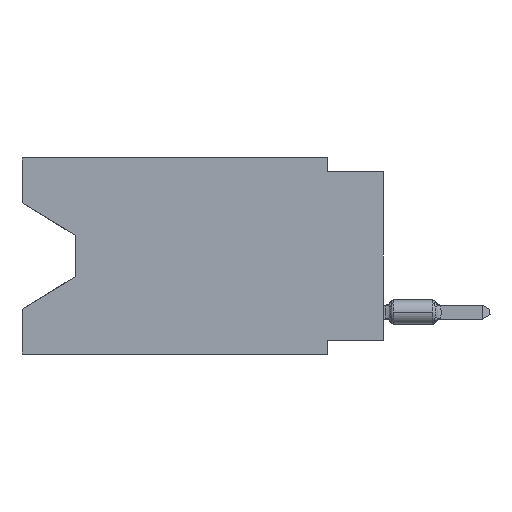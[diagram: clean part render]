
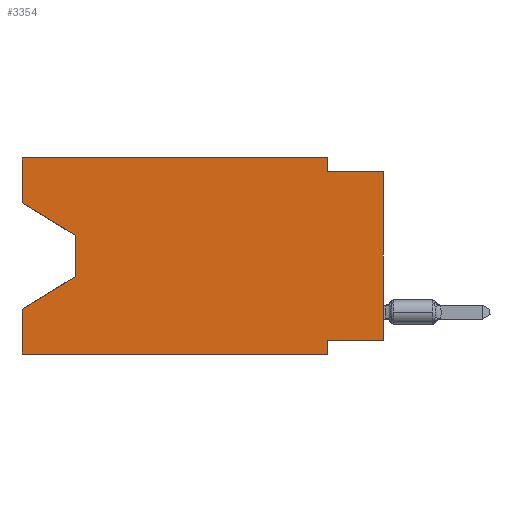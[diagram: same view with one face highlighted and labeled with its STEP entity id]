
A CAD part, left-side view. The second image highlights one B-rep face of the part: STEP entity #3354.
In plain terms, the highlighted planar face has unit normal (-1, 0, 0).
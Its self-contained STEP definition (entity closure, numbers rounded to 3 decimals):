
#882 = VECTOR ( 'NONE', #29066, 1000. ) ;
#1395 = EDGE_CURVE ( 'NONE', #20699, #27107, #30198, .T. ) ;
#1419 = ORIENTED_EDGE ( 'NONE', *, *, #2789, .F. ) ;
#1653 = LINE ( 'NONE', #13884, #13133 ) ;
#1736 = CARTESIAN_POINT ( 'NONE',  ( 0., 2.54, -0.635 ) ) ;
#1854 = LINE ( 'NONE', #32588, #13533 ) ;
#1899 = LINE ( 'NONE', #15554, #28953 ) ;
#2061 = ORIENTED_EDGE ( 'NONE', *, *, #4512, .F. ) ;
#2565 = DIRECTION ( 'NONE',  ( 1., 0., 0. ) ) ;
#2714 = CARTESIAN_POINT ( 'NONE',  ( 0., 0., -0.635 ) ) ;
#2789 = EDGE_CURVE ( 'NONE', #31242, #11664, #1653, .T. ) ;
#2915 = LINE ( 'NONE', #20653, #27316 ) ;
#3056 = VECTOR ( 'NONE', #32800, 1000. ) ;
#3354 = ADVANCED_FACE ( 'NONE', ( #17785 ), #18114, .F. ) ;
#3499 = DIRECTION ( 'NONE',  ( 0., 0., -1. ) ) ;
#4157 = LINE ( 'NONE', #27389, #8981 ) ;
#4435 = VECTOR ( 'NONE', #26715, 1000. ) ;
#4512 = EDGE_CURVE ( 'NONE', #12532, #10847, #24227, .T. ) ;
#4603 = EDGE_CURVE ( 'NONE', #31242, #10847, #4157, .T. ) ;
#4754 = ORIENTED_EDGE ( 'NONE', *, *, #28052, .T. ) ;
#5569 = DIRECTION ( 'NONE',  ( 0., -1., 0. ) ) ;
#5721 = ORIENTED_EDGE ( 'NONE', *, *, #10851, .F. ) ;
#6945 = CARTESIAN_POINT ( 'NONE',  ( 0., 2.54, -8.255 ) ) ;
#7302 = CARTESIAN_POINT ( 'NONE',  ( 0., 16.383, -2.038 ) ) ;
#7756 = VECTOR ( 'NONE', #5569, 1000. ) ;
#7811 = VERTEX_POINT ( 'NONE', #23915 ) ;
#7846 = AXIS2_PLACEMENT_3D ( 'NONE', #25465, #2565, #22962 ) ;
#7919 = LINE ( 'NONE', #10588, #7756 ) ;
#8477 = ORIENTED_EDGE ( 'NONE', *, *, #12286, .T. ) ;
#8686 = CARTESIAN_POINT ( 'NONE',  ( 0., 2.54, -8.89 ) ) ;
#8769 = CARTESIAN_POINT ( 'NONE',  ( 0., 0., -8.255 ) ) ;
#8981 = VECTOR ( 'NONE', #22223, 1000. ) ;
#10149 = CARTESIAN_POINT ( 'NONE',  ( 0., 13.97, -3.505 ) ) ;
#10588 = CARTESIAN_POINT ( 'NONE',  ( 0., 16.383, 0. ) ) ;
#10847 = VERTEX_POINT ( 'NONE', #28151 ) ;
#10851 = EDGE_CURVE ( 'NONE', #13997, #21057, #7919, .T. ) ;
#11664 = VERTEX_POINT ( 'NONE', #26021 ) ;
#12047 = DIRECTION ( 'NONE',  ( 0., 1., 0. ) ) ;
#12245 = EDGE_LOOP ( 'NONE', ( #18997, #8477, #4754, #1419, #19494, #2061, #27753, #27325, #24503, #21351, #5721, #24466 ) ) ;
#12286 = EDGE_CURVE ( 'NONE', #27107, #7811, #30690, .T. ) ;
#12427 = CARTESIAN_POINT ( 'NONE',  ( 0., 16.383, 0. ) ) ;
#12532 = VERTEX_POINT ( 'NONE', #6945 ) ;
#13133 = VECTOR ( 'NONE', #32225, 1000. ) ;
#13533 = VECTOR ( 'NONE', #12047, 1000. ) ;
#13884 = CARTESIAN_POINT ( 'NONE',  ( 0., 16.383, 0. ) ) ;
#13997 = VERTEX_POINT ( 'NONE', #19701 ) ;
#15115 = LINE ( 'NONE', #12427, #3056 ) ;
#15554 = CARTESIAN_POINT ( 'NONE',  ( 0., 2.54, 0. ) ) ;
#15603 = CARTESIAN_POINT ( 'NONE',  ( 0., 16.383, -2.038 ) ) ;
#15651 = DIRECTION ( 'NONE',  ( 0., -0.855, -0.519 ) ) ;
#15811 = CARTESIAN_POINT ( 'NONE',  ( 0., 13.97, -3.505 ) ) ;
#16532 = CARTESIAN_POINT ( 'NONE',  ( 0., 13.97, -5.385 ) ) ;
#17785 = FACE_OUTER_BOUND ( 'NONE', #12245, .T. ) ;
#18058 = EDGE_CURVE ( 'NONE', #31320, #30253, #2915, .T. ) ;
#18114 = PLANE ( 'NONE',  #7846 ) ;
#18171 = DIRECTION ( 'NONE',  ( 0., 0., -1. ) ) ;
#18304 = EDGE_CURVE ( 'NONE', #21057, #31320, #1899, .T. ) ;
#18997 = ORIENTED_EDGE ( 'NONE', *, *, #1395, .T. ) ;
#19494 = ORIENTED_EDGE ( 'NONE', *, *, #4603, .T. ) ;
#19701 = CARTESIAN_POINT ( 'NONE',  ( 0., 16.383, 0. ) ) ;
#20653 = CARTESIAN_POINT ( 'NONE',  ( 0., 0., -0.635 ) ) ;
#20676 = EDGE_CURVE ( 'NONE', #20699, #13997, #15115, .T. ) ;
#20699 = VERTEX_POINT ( 'NONE', #15603 ) ;
#21057 = VERTEX_POINT ( 'NONE', #32931 ) ;
#21351 = ORIENTED_EDGE ( 'NONE', *, *, #18304, .F. ) ;
#21388 = CARTESIAN_POINT ( 'NONE',  ( 0., 0., 0. ) ) ;
#22223 = DIRECTION ( 'NONE',  ( 0., -1., 0. ) ) ;
#22962 = DIRECTION ( 'NONE',  ( 0., 0., -1. ) ) ;
#23915 = CARTESIAN_POINT ( 'NONE',  ( 0., 13.97, -5.385 ) ) ;
#24227 = LINE ( 'NONE', #8686, #30332 ) ;
#24238 = EDGE_CURVE ( 'NONE', #27223, #12532, #1854, .T. ) ;
#24466 = ORIENTED_EDGE ( 'NONE', *, *, #20676, .F. ) ;
#24503 = ORIENTED_EDGE ( 'NONE', *, *, #18058, .F. ) ;
#24687 = LINE ( 'NONE', #16532, #4435 ) ;
#25465 = CARTESIAN_POINT ( 'NONE',  ( 0., 16.383, 0. ) ) ;
#25561 = EDGE_CURVE ( 'NONE', #27223, #30253, #27042, .T. ) ;
#25998 = CARTESIAN_POINT ( 'NONE',  ( 0., 16.383, -8.89 ) ) ;
#26021 = CARTESIAN_POINT ( 'NONE',  ( 0., 16.383, -6.852 ) ) ;
#26715 = DIRECTION ( 'NONE',  ( 0., 0.855, -0.519 ) ) ;
#27042 = LINE ( 'NONE', #21388, #882 ) ;
#27107 = VERTEX_POINT ( 'NONE', #15811 ) ;
#27223 = VERTEX_POINT ( 'NONE', #8769 ) ;
#27316 = VECTOR ( 'NONE', #31161, 1000. ) ;
#27325 = ORIENTED_EDGE ( 'NONE', *, *, #25561, .T. ) ;
#27389 = CARTESIAN_POINT ( 'NONE',  ( 0., 16.383, -8.89 ) ) ;
#27753 = ORIENTED_EDGE ( 'NONE', *, *, #24238, .F. ) ;
#28052 = EDGE_CURVE ( 'NONE', #7811, #11664, #24687, .T. ) ;
#28151 = CARTESIAN_POINT ( 'NONE',  ( 0., 2.54, -8.89 ) ) ;
#28577 = VECTOR ( 'NONE', #18171, 1000. ) ;
#28953 = VECTOR ( 'NONE', #30427, 1000. ) ;
#29066 = DIRECTION ( 'NONE',  ( 0., 0., 1. ) ) ;
#30198 = LINE ( 'NONE', #7302, #33042 ) ;
#30253 = VERTEX_POINT ( 'NONE', #2714 ) ;
#30332 = VECTOR ( 'NONE', #3499, 1000. ) ;
#30427 = DIRECTION ( 'NONE',  ( 0., 0., -1. ) ) ;
#30690 = LINE ( 'NONE', #10149, #28577 ) ;
#31161 = DIRECTION ( 'NONE',  ( 0., -1., 0. ) ) ;
#31242 = VERTEX_POINT ( 'NONE', #25998 ) ;
#31320 = VERTEX_POINT ( 'NONE', #1736 ) ;
#32225 = DIRECTION ( 'NONE',  ( 0., 0., 1. ) ) ;
#32588 = CARTESIAN_POINT ( 'NONE',  ( 0., 0., -8.255 ) ) ;
#32800 = DIRECTION ( 'NONE',  ( 0., 0., 1. ) ) ;
#32931 = CARTESIAN_POINT ( 'NONE',  ( 0., 2.54, 0. ) ) ;
#33042 = VECTOR ( 'NONE', #15651, 1000. ) ;
